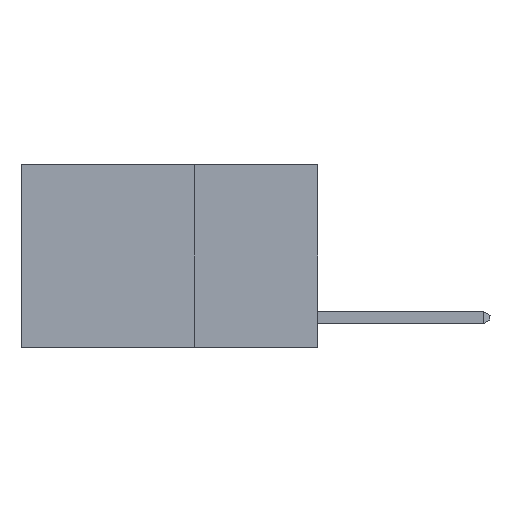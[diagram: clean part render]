
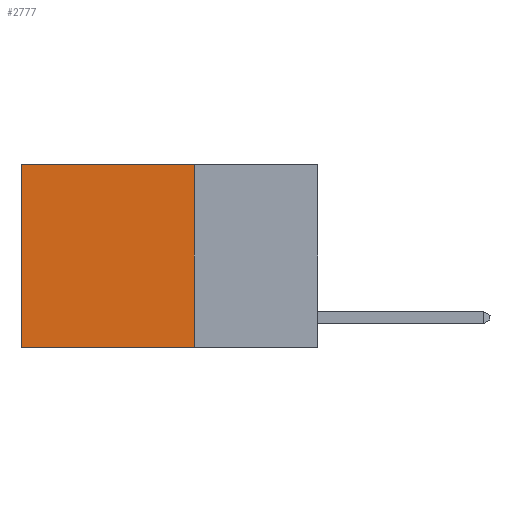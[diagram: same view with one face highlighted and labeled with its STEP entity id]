
A CAD part, left-side view. The second image highlights one B-rep face of the part: STEP entity #2777.
In plain terms, the highlighted planar face has unit normal (-1, 0, 0).
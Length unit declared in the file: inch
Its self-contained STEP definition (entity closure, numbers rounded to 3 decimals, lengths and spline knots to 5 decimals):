
#622 = VECTOR ( 'NONE', #1509, 39.37008 ) ;
#1236 = LINE ( 'NONE', #20013, #15907 ) ;
#1509 = DIRECTION ( 'NONE',  ( 0., 0., -1. ) ) ;
#2777 = ADVANCED_FACE ( 'NONE', ( #23339 ), #19615, .F. ) ;
#3622 = CARTESIAN_POINT ( 'NONE',  ( 0.2625, 0.6, 0. ) ) ;
#3709 = CARTESIAN_POINT ( 'NONE',  ( 0.2625, 0.25, 0. ) ) ;
#4006 = EDGE_LOOP ( 'NONE', ( #23276, #5629, #8658, #10041 ) ) ;
#5567 = DIRECTION ( 'NONE',  ( 0., 0., -1. ) ) ;
#5629 = ORIENTED_EDGE ( 'NONE', *, *, #17353, .F. ) ;
#5810 = LINE ( 'NONE', #18726, #622 ) ;
#6715 = DIRECTION ( 'NONE',  ( 0., 1., 0. ) ) ;
#7096 = EDGE_CURVE ( 'NONE', #20791, #16034, #14476, .T. ) ;
#8262 = EDGE_CURVE ( 'NONE', #20095, #20603, #5810, .T. ) ;
#8658 = ORIENTED_EDGE ( 'NONE', *, *, #8262, .F. ) ;
#9706 = LINE ( 'NONE', #3709, #23705 ) ;
#10041 = ORIENTED_EDGE ( 'NONE', *, *, #16991, .T. ) ;
#11394 = DIRECTION ( 'NONE',  ( 0., 1., 0. ) ) ;
#12066 = DIRECTION ( 'NONE',  ( 0., 0., -1. ) ) ;
#14476 = LINE ( 'NONE', #3622, #24010 ) ;
#15907 = VECTOR ( 'NONE', #6715, 39.37008 ) ;
#16034 = VERTEX_POINT ( 'NONE', #19584 ) ;
#16576 = CARTESIAN_POINT ( 'NONE',  ( 0.2625, 0.25, 0. ) ) ;
#16991 = EDGE_CURVE ( 'NONE', #20095, #20791, #9706, .T. ) ;
#17353 = EDGE_CURVE ( 'NONE', #20603, #16034, #1236, .T. ) ;
#18397 = CARTESIAN_POINT ( 'NONE',  ( 0.2625, 0.6, 0. ) ) ;
#18726 = CARTESIAN_POINT ( 'NONE',  ( 0.2625, 0.25, 0. ) ) ;
#19584 = CARTESIAN_POINT ( 'NONE',  ( 0.2625, 0.6, -0.37 ) ) ;
#19615 = PLANE ( 'NONE',  #21672 ) ;
#19665 = CARTESIAN_POINT ( 'NONE',  ( 0.2625, 0.25, -0.37 ) ) ;
#20013 = CARTESIAN_POINT ( 'NONE',  ( 0.2625, 0.25, -0.37 ) ) ;
#20095 = VERTEX_POINT ( 'NONE', #16576 ) ;
#20603 = VERTEX_POINT ( 'NONE', #19665 ) ;
#20791 = VERTEX_POINT ( 'NONE', #18397 ) ;
#21512 = CARTESIAN_POINT ( 'NONE',  ( 0.2625, 0.25, 0. ) ) ;
#21672 = AXIS2_PLACEMENT_3D ( 'NONE', #21512, #23451, #12066 ) ;
#23276 = ORIENTED_EDGE ( 'NONE', *, *, #7096, .T. ) ;
#23339 = FACE_OUTER_BOUND ( 'NONE', #4006, .T. ) ;
#23451 = DIRECTION ( 'NONE',  ( 1., 0., 0. ) ) ;
#23705 = VECTOR ( 'NONE', #11394, 39.37008 ) ;
#24010 = VECTOR ( 'NONE', #5567, 39.37008 ) ;
